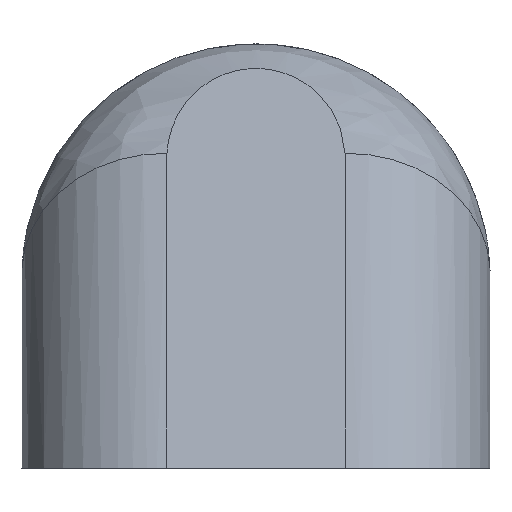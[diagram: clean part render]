
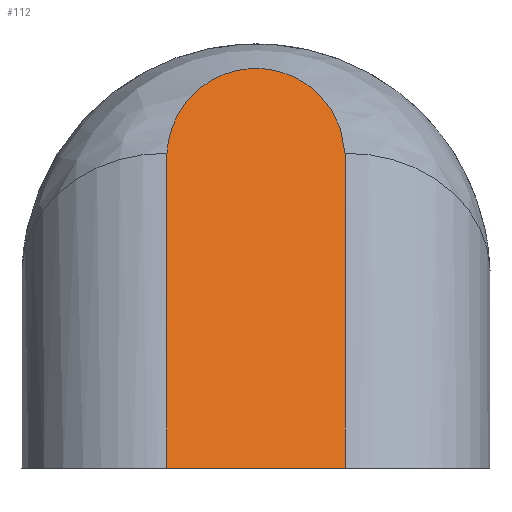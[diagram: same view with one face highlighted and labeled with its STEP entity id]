
A CAD part, left-side view. The second image highlights one B-rep face of the part: STEP entity #112.
In plain terms, the highlighted planar face has unit normal (-0.557, 0, 0.83).
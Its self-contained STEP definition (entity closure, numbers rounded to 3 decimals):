
#10 = CARTESIAN_POINT ( 'NONE',  ( -75.43, 55.484, -4.003 ) ) ;
#94 =( BOUNDED_CURVE ( )  B_SPLINE_CURVE ( 3, ( #159, #153, #151, #149 ),
 .UNSPECIFIED., .F., .F. ) 
 B_SPLINE_CURVE_WITH_KNOTS ( ( 4, 4 ),
 ( 1.62, 4.664 ),
 .UNSPECIFIED. ) 
 CURVE ( )  GEOMETRIC_REPRESENTATION_ITEM ( )  RATIONAL_B_SPLINE_CURVE ( ( 1., 0.366, 0.366, 1. ) ) 
 REPRESENTATION_ITEM ( '' )  );
#112 = ADVANCED_FACE ( 'NONE', ( #426 ), #556, .T. ) ;
#114 = DIRECTION ( 'NONE',  ( -0.83, 0., -0.557 ) ) ;
#116 = DIRECTION ( 'NONE',  ( -0.557, 0., 0.83 ) ) ;
#145 = CARTESIAN_POINT ( 'NONE',  ( -75.43, 62.541, -4.003 ) ) ;
#146 = DIRECTION ( 'NONE',  ( 0., -1., 0. ) ) ;
#149 = CARTESIAN_POINT ( 'NONE',  ( -38.203, 69.617, 20.974 ) ) ;
#151 = CARTESIAN_POINT ( 'NONE',  ( -19.031, 68.99, 33.837 ) ) ;
#152 = CARTESIAN_POINT ( 'NONE',  ( -81.313, 55.484, -7.95 ) ) ;
#153 = CARTESIAN_POINT ( 'NONE',  ( -19.031, 56.111, 33.837 ) ) ;
#154 = DIRECTION ( 'NONE',  ( 0.83, 0., 0.557 ) ) ;
#159 = CARTESIAN_POINT ( 'NONE',  ( -38.203, 55.484, 20.974 ) ) ;
#196 = CARTESIAN_POINT ( 'NONE',  ( -38.203, 55.484, 20.974 ) ) ;
#199 = EDGE_CURVE ( 'NONE', #614, #516, #383, .T. ) ;
#248 = VECTOR ( 'NONE', #146, 1000. ) ;
#250 = VECTOR ( 'NONE', #154, 1000. ) ;
#254 = LINE ( 'NONE', #145, #248 ) ;
#260 = LINE ( 'NONE', #152, #250 ) ;
#274 = CARTESIAN_POINT ( 'NONE',  ( -75.43, 69.617, -4.003 ) ) ;
#379 = VECTOR ( 'NONE', #627, 1000. ) ;
#383 = LINE ( 'NONE', #636, #379 ) ;
#426 = FACE_OUTER_BOUND ( 'NONE', #740, .T. ) ;
#516 = VERTEX_POINT ( 'NONE', #274 ) ;
#527 = ORIENTED_EDGE ( 'NONE', *, *, #199, .T. ) ;
#529 = CARTESIAN_POINT ( 'NONE',  ( -81.313, 62.541, -7.95 ) ) ;
#556 = PLANE ( 'NONE',  #742 ) ;
#614 = VERTEX_POINT ( 'NONE', #825 ) ;
#627 = DIRECTION ( 'NONE',  ( -0.83, 0., -0.557 ) ) ;
#636 = CARTESIAN_POINT ( 'NONE',  ( -81.313, 69.617, -7.95 ) ) ;
#689 = VERTEX_POINT ( 'NONE', #10 ) ;
#720 = ORIENTED_EDGE ( 'NONE', *, *, #947, .T. ) ;
#740 = EDGE_LOOP ( 'NONE', ( #527, #720, #813, #949 ) ) ;
#742 = AXIS2_PLACEMENT_3D ( 'NONE', #529, #116, #114 ) ;
#813 = ORIENTED_EDGE ( 'NONE', *, *, #936, .T. ) ;
#824 = VERTEX_POINT ( 'NONE', #196 ) ;
#825 = CARTESIAN_POINT ( 'NONE',  ( -38.203, 69.617, 20.974 ) ) ;
#931 = EDGE_CURVE ( 'NONE', #824, #614, #94, .T. ) ;
#936 = EDGE_CURVE ( 'NONE', #689, #824, #260, .T. ) ;
#947 = EDGE_CURVE ( 'NONE', #516, #689, #254, .T. ) ;
#949 = ORIENTED_EDGE ( 'NONE', *, *, #931, .T. ) ;
